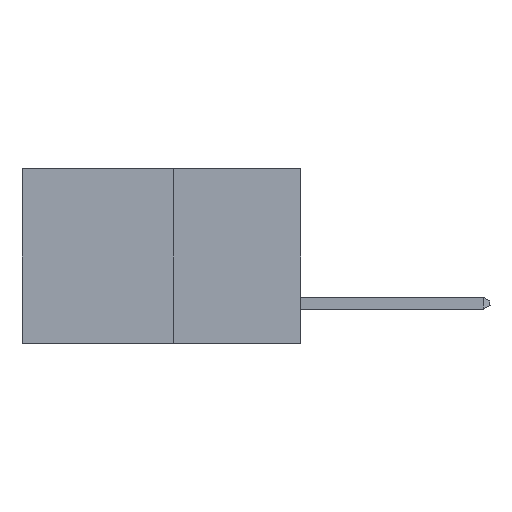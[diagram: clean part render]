
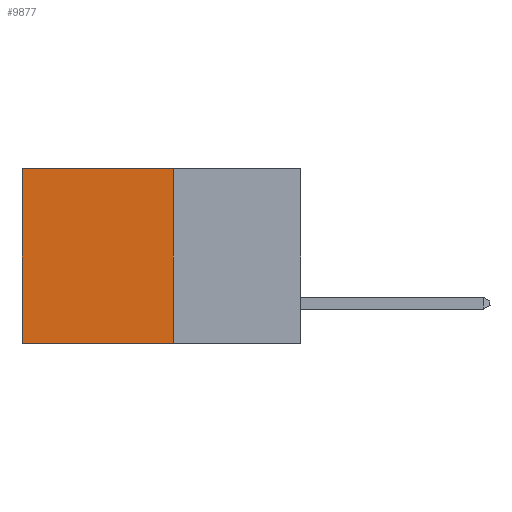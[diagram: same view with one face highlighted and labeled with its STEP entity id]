
A CAD part, left-side view. The second image highlights one B-rep face of the part: STEP entity #9877.
In plain terms, the highlighted planar face has unit normal (-1, 0, 0).
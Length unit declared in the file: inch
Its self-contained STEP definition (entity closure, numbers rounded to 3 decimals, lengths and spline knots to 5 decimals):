
#11 = ORIENTED_EDGE ( 'NONE', *, *, #8907, .T. ) ;
#1705 = CARTESIAN_POINT ( 'NONE',  ( 0.277, 0.27, -0.37 ) ) ;
#1835 = DIRECTION ( 'NONE',  ( 1., 0., 0. ) ) ;
#1983 = DIRECTION ( 'NONE',  ( 0., 1., 0. ) ) ;
#1985 = LINE ( 'NONE', #9586, #12536 ) ;
#2168 = CARTESIAN_POINT ( 'NONE',  ( 0.277, 0.59, -0.37 ) ) ;
#2477 = DIRECTION ( 'NONE',  ( 0., 0., -1. ) ) ;
#2973 = VERTEX_POINT ( 'NONE', #6281 ) ;
#3136 = CARTESIAN_POINT ( 'NONE',  ( 0.277, 0.59, 0. ) ) ;
#3246 = VECTOR ( 'NONE', #1983, 39.37008 ) ;
#4405 = CARTESIAN_POINT ( 'NONE',  ( 0.277, 0.27, -0.37 ) ) ;
#4809 = EDGE_CURVE ( 'NONE', #5247, #8773, #6019, .T. ) ;
#5247 = VERTEX_POINT ( 'NONE', #4405 ) ;
#5662 = AXIS2_PLACEMENT_3D ( 'NONE', #8012, #1835, #9041 ) ;
#5993 = LINE ( 'NONE', #12992, #8662 ) ;
#6007 = PLANE ( 'NONE',  #5662 ) ;
#6019 = LINE ( 'NONE', #1705, #3246 ) ;
#6281 = CARTESIAN_POINT ( 'NONE',  ( 0.277, 0.27, 0. ) ) ;
#6329 = EDGE_CURVE ( 'NONE', #9203, #8773, #5993, .T. ) ;
#6458 = EDGE_LOOP ( 'NONE', ( #7807, #7497, #8429, #11 ) ) ;
#7384 = LINE ( 'NONE', #8627, #13019 ) ;
#7497 = ORIENTED_EDGE ( 'NONE', *, *, #4809, .F. ) ;
#7675 = EDGE_CURVE ( 'NONE', #2973, #5247, #7384, .T. ) ;
#7807 = ORIENTED_EDGE ( 'NONE', *, *, #6329, .T. ) ;
#8012 = CARTESIAN_POINT ( 'NONE',  ( 0.277, 0.27, -0.37 ) ) ;
#8247 = FACE_OUTER_BOUND ( 'NONE', #6458, .T. ) ;
#8429 = ORIENTED_EDGE ( 'NONE', *, *, #7675, .F. ) ;
#8627 = CARTESIAN_POINT ( 'NONE',  ( 0.277, 0.27, -0.37 ) ) ;
#8662 = VECTOR ( 'NONE', #12425, 39.37008 ) ;
#8773 = VERTEX_POINT ( 'NONE', #2168 ) ;
#8907 = EDGE_CURVE ( 'NONE', #2973, #9203, #1985, .T. ) ;
#9041 = DIRECTION ( 'NONE',  ( 0., 0., -1. ) ) ;
#9203 = VERTEX_POINT ( 'NONE', #3136 ) ;
#9586 = CARTESIAN_POINT ( 'NONE',  ( 0.277, 0.27, 0. ) ) ;
#9877 = ADVANCED_FACE ( 'NONE', ( #8247 ), #6007, .F. ) ;
#10557 = DIRECTION ( 'NONE',  ( 0., 1., 0. ) ) ;
#12425 = DIRECTION ( 'NONE',  ( 0., 0., -1. ) ) ;
#12536 = VECTOR ( 'NONE', #10557, 39.37008 ) ;
#12992 = CARTESIAN_POINT ( 'NONE',  ( 0.277, 0.59, -0.37 ) ) ;
#13019 = VECTOR ( 'NONE', #2477, 39.37008 ) ;
